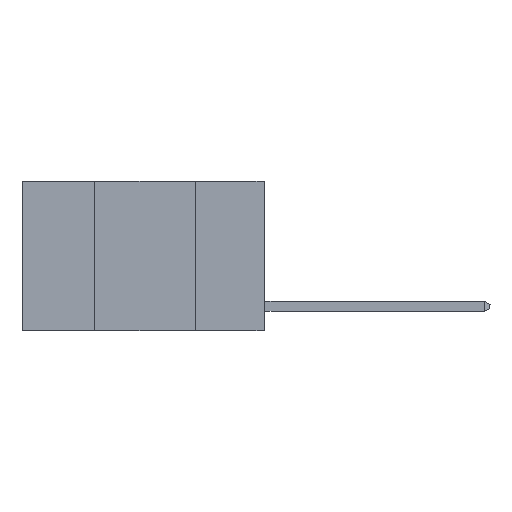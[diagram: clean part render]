
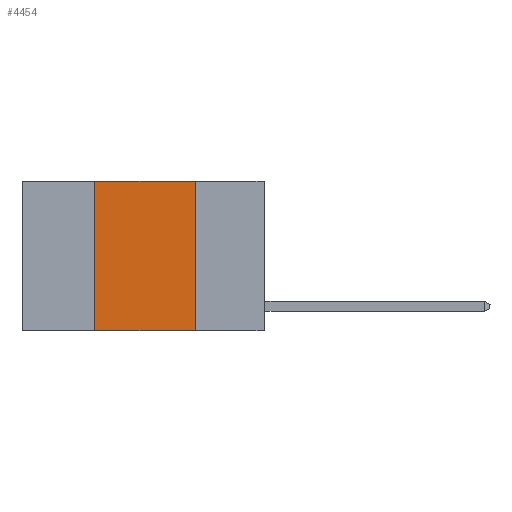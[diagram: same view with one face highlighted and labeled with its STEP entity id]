
A CAD part, left-side view. The second image highlights one B-rep face of the part: STEP entity #4454.
In plain terms, the highlighted planar face has unit normal (-1, 0, 0).
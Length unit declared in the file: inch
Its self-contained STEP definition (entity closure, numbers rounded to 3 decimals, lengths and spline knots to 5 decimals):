
#69 = CARTESIAN_POINT ( 'NONE',  ( 0., 0.6, -0.37 ) ) ;
#987 = VECTOR ( 'NONE', #14535, 39.37008 ) ;
#1474 = DIRECTION ( 'NONE',  ( 0., 0., -1. ) ) ;
#3928 = CARTESIAN_POINT ( 'NONE',  ( 0., 0.17, 0. ) ) ;
#4038 = CARTESIAN_POINT ( 'NONE',  ( 0., 0.42, 0. ) ) ;
#4132 = PLANE ( 'NONE',  #17570 ) ;
#4454 = ADVANCED_FACE ( 'NONE', ( #10274 ), #4132, .F. ) ;
#5221 = CARTESIAN_POINT ( 'NONE',  ( 0., 0.6, 0. ) ) ;
#5641 = DIRECTION ( 'NONE',  ( 0., 0., -1. ) ) ;
#6347 = VERTEX_POINT ( 'NONE', #7860 ) ;
#6690 = EDGE_CURVE ( 'NONE', #22124, #6347, #23229, .T. ) ;
#7547 = VERTEX_POINT ( 'NONE', #4038 ) ;
#7664 = CARTESIAN_POINT ( 'NONE',  ( 0., 0.6, 0. ) ) ;
#7748 = ORIENTED_EDGE ( 'NONE', *, *, #22798, .F. ) ;
#7860 = CARTESIAN_POINT ( 'NONE',  ( 0., 0.17, -0.37 ) ) ;
#9185 = CARTESIAN_POINT ( 'NONE',  ( 0., 0.42, -0.37 ) ) ;
#10138 = EDGE_LOOP ( 'NONE', ( #7748, #15088, #23014, #14201 ) ) ;
#10274 = FACE_OUTER_BOUND ( 'NONE', #10138, .T. ) ;
#10476 = EDGE_CURVE ( 'NONE', #7547, #20318, #16179, .T. ) ;
#10589 = VECTOR ( 'NONE', #1474, 39.37008 ) ;
#10945 = DIRECTION ( 'NONE',  ( 1., 0., 0. ) ) ;
#14201 = ORIENTED_EDGE ( 'NONE', *, *, #6690, .T. ) ;
#14535 = DIRECTION ( 'NONE',  ( 0., -1., 0. ) ) ;
#14668 = DIRECTION ( 'NONE',  ( 0., -1., 0. ) ) ;
#15088 = ORIENTED_EDGE ( 'NONE', *, *, #10476, .F. ) ;
#15777 = DIRECTION ( 'NONE',  ( 0., 0., 1. ) ) ;
#16179 = LINE ( 'NONE', #5221, #987 ) ;
#16188 = VECTOR ( 'NONE', #14668, 39.37008 ) ;
#17325 = LINE ( 'NONE', #22934, #22891 ) ;
#17570 = AXIS2_PLACEMENT_3D ( 'NONE', #7664, #10945, #5641 ) ;
#17619 = CARTESIAN_POINT ( 'NONE',  ( 0., 0.17, 0. ) ) ;
#18936 = EDGE_CURVE ( 'NONE', #22124, #7547, #17325, .T. ) ;
#20318 = VERTEX_POINT ( 'NONE', #3928 ) ;
#21266 = LINE ( 'NONE', #17619, #10589 ) ;
#22124 = VERTEX_POINT ( 'NONE', #9185 ) ;
#22798 = EDGE_CURVE ( 'NONE', #20318, #6347, #21266, .T. ) ;
#22891 = VECTOR ( 'NONE', #15777, 39.37008 ) ;
#22934 = CARTESIAN_POINT ( 'NONE',  ( 0., 0.42, 0. ) ) ;
#23014 = ORIENTED_EDGE ( 'NONE', *, *, #18936, .F. ) ;
#23229 = LINE ( 'NONE', #69, #16188 ) ;
